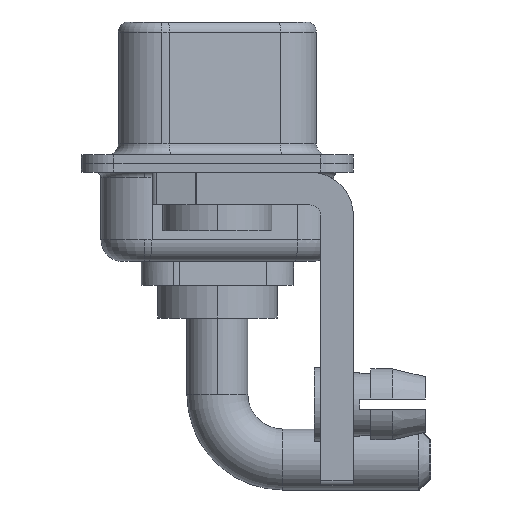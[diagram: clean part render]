
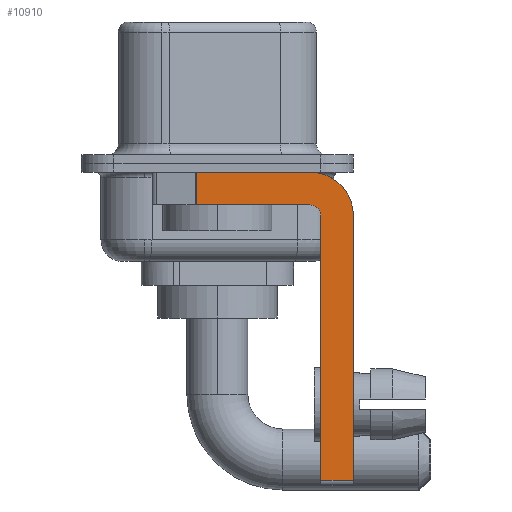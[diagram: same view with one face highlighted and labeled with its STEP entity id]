
A CAD part, left-side view. The second image highlights one B-rep face of the part: STEP entity #10910.
In plain terms, the highlighted planar face has unit normal (-1, 0, 0).
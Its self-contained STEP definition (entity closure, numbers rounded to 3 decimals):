
#10 = LINE ( 'NONE', #15668, #148 ) ;
#148 = VECTOR ( 'NONE', #9177, 1000. ) ;
#211 = EDGE_CURVE ( 'NONE', #6987, #4506, #7202, .T. ) ;
#315 = EDGE_CURVE ( 'NONE', #474, #15103, #14872, .T. ) ;
#474 = VERTEX_POINT ( 'NONE', #2123 ) ;
#952 = CARTESIAN_POINT ( 'NONE',  ( -2.9, -4.75, -14.8 ) ) ;
#1029 = DIRECTION ( 'NONE',  ( 0., 1., 0. ) ) ;
#1155 = ORIENTED_EDGE ( 'NONE', *, *, #3520, .F. ) ;
#1396 = DIRECTION ( 'NONE',  ( 1., 0., 0. ) ) ;
#2103 = CARTESIAN_POINT ( 'NONE',  ( -2.9, -4.25, -2.4 ) ) ;
#2123 = CARTESIAN_POINT ( 'NONE',  ( -2.9, -4.75, -2.4 ) ) ;
#2304 = LINE ( 'NONE', #12729, #15692 ) ;
#3073 = CARTESIAN_POINT ( 'NONE',  ( -2.9, -4.25, -14.55 ) ) ;
#3384 = AXIS2_PLACEMENT_3D ( 'NONE', #2103, #12525, #12275 ) ;
#3520 = EDGE_CURVE ( 'NONE', #14331, #474, #15331, .T. ) ;
#3539 = DIRECTION ( 'NONE',  ( 0., -1., 0. ) ) ;
#3745 = AXIS2_PLACEMENT_3D ( 'NONE', #16724, #1396, #13021 ) ;
#3787 = VERTEX_POINT ( 'NONE', #9660 ) ;
#4506 = VERTEX_POINT ( 'NONE', #9460 ) ;
#5215 = ORIENTED_EDGE ( 'NONE', *, *, #211, .F. ) ;
#5757 = VERTEX_POINT ( 'NONE', #8731 ) ;
#5909 = CARTESIAN_POINT ( 'NONE',  ( -2.9, -4.25, -0.4 ) ) ;
#6439 = DIRECTION ( 'NONE',  ( 0., 0., 1. ) ) ;
#6987 = VERTEX_POINT ( 'NONE', #5909 ) ;
#7090 = EDGE_CURVE ( 'NONE', #15103, #3787, #2304, .T. ) ;
#7202 = CIRCLE ( 'NONE', #3384, 2. ) ;
#7391 = LINE ( 'NONE', #10115, #15161 ) ;
#7645 = PLANE ( 'NONE',  #3745 ) ;
#7899 = EDGE_CURVE ( 'NONE', #5757, #6987, #7391, .T. ) ;
#8299 = ORIENTED_EDGE ( 'NONE', *, *, #7090, .F. ) ;
#8404 = VERTEX_POINT ( 'NONE', #11706 ) ;
#8731 = CARTESIAN_POINT ( 'NONE',  ( -2.9, 0.978, -0.4 ) ) ;
#8898 = CARTESIAN_POINT ( 'NONE',  ( -2.9, -4.25, -1.9 ) ) ;
#8938 = FACE_OUTER_BOUND ( 'NONE', #9186, .T. ) ;
#8967 = DIRECTION ( 'NONE',  ( -1., 0., 0. ) ) ;
#9177 = DIRECTION ( 'NONE',  ( 0., 0., -1. ) ) ;
#9186 = EDGE_LOOP ( 'NONE', ( #13349, #9782, #8299, #16829, #1155, #10140, #16451, #5215 ) ) ;
#9460 = CARTESIAN_POINT ( 'NONE',  ( -2.9, -6.25, -2.4 ) ) ;
#9577 = DIRECTION ( 'NONE',  ( 0., -1., 0. ) ) ;
#9659 = LINE ( 'NONE', #3073, #9703 ) ;
#9660 = CARTESIAN_POINT ( 'NONE',  ( -2.9, 0.978, -1.9 ) ) ;
#9703 = VECTOR ( 'NONE', #9577, 1000. ) ;
#9782 = ORIENTED_EDGE ( 'NONE', *, *, #16066, .T. ) ;
#9914 = CARTESIAN_POINT ( 'NONE',  ( -2.9, -4.75, -14.55 ) ) ;
#9941 = AXIS2_PLACEMENT_3D ( 'NONE', #15629, #8967, #10145 ) ;
#10115 = CARTESIAN_POINT ( 'NONE',  ( -2.9, 3., -0.4 ) ) ;
#10140 = ORIENTED_EDGE ( 'NONE', *, *, #16084, .T. ) ;
#10145 = DIRECTION ( 'NONE',  ( 0., 0., 1. ) ) ;
#10671 = LINE ( 'NONE', #14958, #13221 ) ;
#10910 = ADVANCED_FACE ( 'NONE', ( #8938 ), #7645, .F. ) ;
#11706 = CARTESIAN_POINT ( 'NONE',  ( -2.9, -6.25, -14.55 ) ) ;
#12275 = DIRECTION ( 'NONE',  ( 0., 0., -1. ) ) ;
#12525 = DIRECTION ( 'NONE',  ( 1., 0., 0. ) ) ;
#12729 = CARTESIAN_POINT ( 'NONE',  ( -2.9, -4.25, -1.9 ) ) ;
#12817 = VECTOR ( 'NONE', #6439, 1000. ) ;
#13021 = DIRECTION ( 'NONE',  ( 0., 0., -1. ) ) ;
#13221 = VECTOR ( 'NONE', #15988, 1000. ) ;
#13349 = ORIENTED_EDGE ( 'NONE', *, *, #7899, .F. ) ;
#14331 = VERTEX_POINT ( 'NONE', #9914 ) ;
#14588 = EDGE_CURVE ( 'NONE', #4506, #8404, #10671, .T. ) ;
#14872 = CIRCLE ( 'NONE', #9941, 0.5 ) ;
#14958 = CARTESIAN_POINT ( 'NONE',  ( -2.9, -6.25, -2.4 ) ) ;
#15103 = VERTEX_POINT ( 'NONE', #8898 ) ;
#15161 = VECTOR ( 'NONE', #3539, 1000. ) ;
#15331 = LINE ( 'NONE', #952, #12817 ) ;
#15629 = CARTESIAN_POINT ( 'NONE',  ( -2.9, -4.25, -2.4 ) ) ;
#15668 = CARTESIAN_POINT ( 'NONE',  ( -2.9, 0.978, -1.9 ) ) ;
#15692 = VECTOR ( 'NONE', #1029, 1000. ) ;
#15988 = DIRECTION ( 'NONE',  ( 0., 0., -1. ) ) ;
#16066 = EDGE_CURVE ( 'NONE', #5757, #3787, #10, .T. ) ;
#16084 = EDGE_CURVE ( 'NONE', #14331, #8404, #9659, .T. ) ;
#16451 = ORIENTED_EDGE ( 'NONE', *, *, #14588, .F. ) ;
#16724 = CARTESIAN_POINT ( 'NONE',  ( -2.9, -4.25, -2.4 ) ) ;
#16829 = ORIENTED_EDGE ( 'NONE', *, *, #315, .F. ) ;
